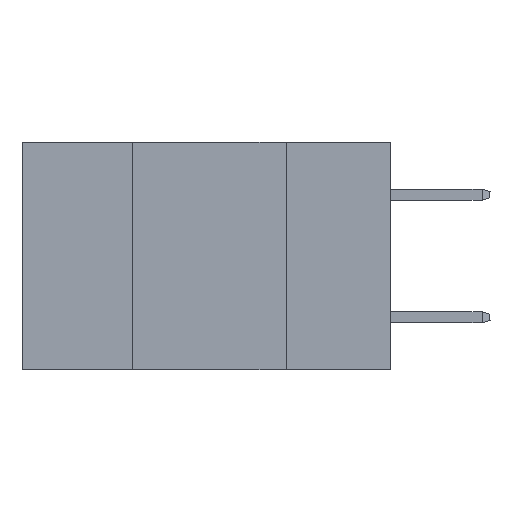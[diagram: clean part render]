
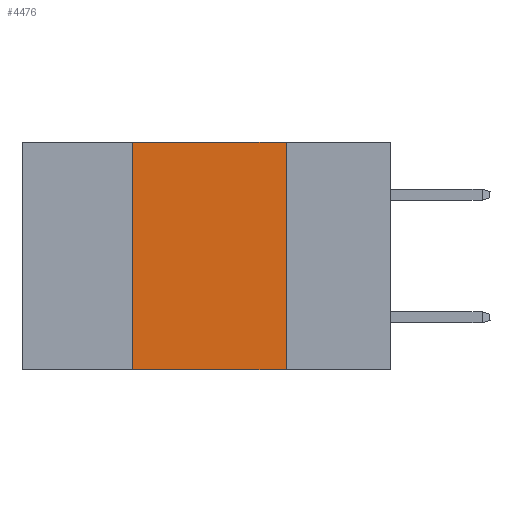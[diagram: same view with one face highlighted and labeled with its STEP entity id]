
A CAD part, left-side view. The second image highlights one B-rep face of the part: STEP entity #4476.
In plain terms, the highlighted planar face has unit normal (-1, 0, 0).
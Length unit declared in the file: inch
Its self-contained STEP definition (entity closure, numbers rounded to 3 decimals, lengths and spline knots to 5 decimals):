
#97 = PLANE ( 'NONE',  #7893 ) ;
#324 = VERTEX_POINT ( 'NONE', #12589 ) ;
#1034 = VECTOR ( 'NONE', #12844, 39.37008 ) ;
#1213 = EDGE_CURVE ( 'NONE', #3396, #2943, #4063, .T. ) ;
#1470 = LINE ( 'NONE', #3978, #13993 ) ;
#2425 = EDGE_CURVE ( 'NONE', #324, #13692, #1470, .T. ) ;
#2943 = VERTEX_POINT ( 'NONE', #7229 ) ;
#2978 = EDGE_CURVE ( 'NONE', #13692, #2943, #7732, .T. ) ;
#3396 = VERTEX_POINT ( 'NONE', #8782 ) ;
#3738 = DIRECTION ( 'NONE',  ( 0., 0., 1. ) ) ;
#3978 = CARTESIAN_POINT ( 'NONE',  ( 0., 0.6, 0. ) ) ;
#4063 = LINE ( 'NONE', #11800, #1034 ) ;
#4092 = ORIENTED_EDGE ( 'NONE', *, *, #2425, .F. ) ;
#4304 = LINE ( 'NONE', #11432, #13069 ) ;
#4476 = ADVANCED_FACE ( 'NONE', ( #12293 ), #97, .F. ) ;
#7229 = CARTESIAN_POINT ( 'NONE',  ( 0., 0.17, -0.37 ) ) ;
#7501 = ORIENTED_EDGE ( 'NONE', *, *, #2978, .F. ) ;
#7732 = LINE ( 'NONE', #12974, #12204 ) ;
#7893 = AXIS2_PLACEMENT_3D ( 'NONE', #9463, #10585, #11722 ) ;
#8204 = DIRECTION ( 'NONE',  ( 0., 0., -1. ) ) ;
#8782 = CARTESIAN_POINT ( 'NONE',  ( 0., 0.42, -0.37 ) ) ;
#9463 = CARTESIAN_POINT ( 'NONE',  ( 0., 0.6, 0. ) ) ;
#10330 = CARTESIAN_POINT ( 'NONE',  ( 0., 0.17, 0. ) ) ;
#10585 = DIRECTION ( 'NONE',  ( 1., 0., 0. ) ) ;
#10959 = DIRECTION ( 'NONE',  ( 0., -1., 0. ) ) ;
#11432 = CARTESIAN_POINT ( 'NONE',  ( 0., 0.42, 0. ) ) ;
#11722 = DIRECTION ( 'NONE',  ( 0., 0., -1. ) ) ;
#11800 = CARTESIAN_POINT ( 'NONE',  ( 0., 0.6, -0.37 ) ) ;
#12204 = VECTOR ( 'NONE', #8204, 39.37008 ) ;
#12270 = ORIENTED_EDGE ( 'NONE', *, *, #13760, .F. ) ;
#12293 = FACE_OUTER_BOUND ( 'NONE', #14093, .T. ) ;
#12589 = CARTESIAN_POINT ( 'NONE',  ( 0., 0.42, 0. ) ) ;
#12844 = DIRECTION ( 'NONE',  ( 0., -1., 0. ) ) ;
#12974 = CARTESIAN_POINT ( 'NONE',  ( 0., 0.17, 0. ) ) ;
#13069 = VECTOR ( 'NONE', #3738, 39.37008 ) ;
#13692 = VERTEX_POINT ( 'NONE', #10330 ) ;
#13760 = EDGE_CURVE ( 'NONE', #3396, #324, #4304, .T. ) ;
#13993 = VECTOR ( 'NONE', #10959, 39.37008 ) ;
#14093 = EDGE_LOOP ( 'NONE', ( #7501, #4092, #12270, #14172 ) ) ;
#14172 = ORIENTED_EDGE ( 'NONE', *, *, #1213, .T. ) ;
